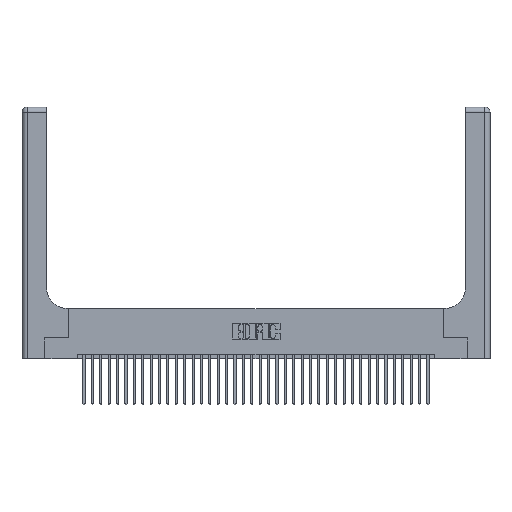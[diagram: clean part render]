
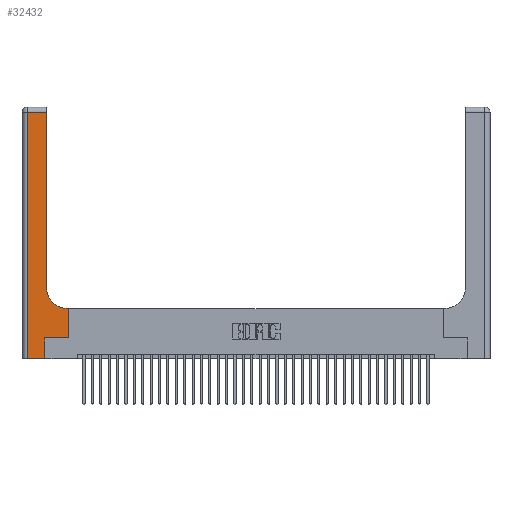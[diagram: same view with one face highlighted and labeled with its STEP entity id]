
A CAD part, top view. The second image highlights one B-rep face of the part: STEP entity #32432.
In plain terms, the highlighted planar face has unit normal (0, 0, 1).
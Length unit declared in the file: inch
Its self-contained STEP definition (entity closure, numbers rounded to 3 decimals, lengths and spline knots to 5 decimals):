
#152 = CARTESIAN_POINT ( 'NONE',  ( 0.5585, 0.6, 0.37 ) ) ;
#202 = LINE ( 'NONE', #612, #22885 ) ;
#358 = EDGE_CURVE ( 'NONE', #30124, #27426, #10339, .T. ) ;
#612 = CARTESIAN_POINT ( 'NONE',  ( 0.269, 0.25, 0.37 ) ) ;
#857 = ORIENTED_EDGE ( 'NONE', *, *, #20001, .T. ) ;
#1382 = FACE_OUTER_BOUND ( 'NONE', #37550, .T. ) ;
#1496 = VERTEX_POINT ( 'NONE', #13183 ) ;
#1788 = CARTESIAN_POINT ( 'NONE',  ( 0.269, 0., 0.37 ) ) ;
#1844 = VERTEX_POINT ( 'NONE', #35211 ) ;
#2411 = VECTOR ( 'NONE', #21373, 39.37008 ) ;
#2478 = VECTOR ( 'NONE', #8937, 39.37008 ) ;
#2539 = CARTESIAN_POINT ( 'NONE',  ( 0.269, 0., 0.37 ) ) ;
#2975 = CARTESIAN_POINT ( 'NONE',  ( 0.06, 0., 0.37 ) ) ;
#3069 = VERTEX_POINT ( 'NONE', #37576 ) ;
#3106 = VERTEX_POINT ( 'NONE', #2539 ) ;
#3187 = VECTOR ( 'NONE', #6990, 39.37008 ) ;
#3831 = EDGE_CURVE ( 'NONE', #27426, #3106, #36082, .T. ) ;
#3844 = VERTEX_POINT ( 'NONE', #32644 ) ;
#3907 = LINE ( 'NONE', #16998, #26511 ) ;
#4087 = ORIENTED_EDGE ( 'NONE', *, *, #19278, .T. ) ;
#5732 = VECTOR ( 'NONE', #6165, 39.37008 ) ;
#6165 = DIRECTION ( 'NONE',  ( 1., 0., 0. ) ) ;
#6990 = DIRECTION ( 'NONE',  ( 0., 1., 0. ) ) ;
#7220 = EDGE_CURVE ( 'NONE', #1844, #3069, #20760, .T. ) ;
#7291 = EDGE_CURVE ( 'NONE', #34413, #14493, #32674, .T. ) ;
#7973 = PLANE ( 'NONE',  #26061 ) ;
#8937 = DIRECTION ( 'NONE',  ( -1., 0., 0. ) ) ;
#9206 = ORIENTED_EDGE ( 'NONE', *, *, #7291, .T. ) ;
#9554 = CARTESIAN_POINT ( 'NONE',  ( 0.06, 3., 0.37 ) ) ;
#10091 = ORIENTED_EDGE ( 'NONE', *, *, #21156, .T. ) ;
#10339 = LINE ( 'NONE', #9554, #2411 ) ;
#10768 = DIRECTION ( 'NONE',  ( 0., 0., -1. ) ) ;
#10820 = CARTESIAN_POINT ( 'NONE',  ( 0., 3., 0.37 ) ) ;
#10959 = DIRECTION ( 'NONE',  ( 0., 0., -1. ) ) ;
#13183 = CARTESIAN_POINT ( 'NONE',  ( 0.269, 0.25, 0.37 ) ) ;
#13193 = DIRECTION ( 'NONE',  ( -1., 0., 0. ) ) ;
#14493 = VERTEX_POINT ( 'NONE', #30005 ) ;
#16546 = DIRECTION ( 'NONE',  ( 0., 1., 0. ) ) ;
#16998 = CARTESIAN_POINT ( 'NONE',  ( 0.5585, 0.25, 0.37 ) ) ;
#17054 = VECTOR ( 'NONE', #13193, 39.37008 ) ;
#18568 = CARTESIAN_POINT ( 'NONE',  ( 0.2915, 3., 0.37 ) ) ;
#18683 = CARTESIAN_POINT ( 'NONE',  ( 0.06, 2.94, 0.37 ) ) ;
#19200 = VECTOR ( 'NONE', #16546, 39.37008 ) ;
#19278 = EDGE_CURVE ( 'NONE', #3106, #1496, #21985, .T. ) ;
#20001 = EDGE_CURVE ( 'NONE', #3844, #34413, #3907, .T. ) ;
#20760 = LINE ( 'NONE', #18568, #3187 ) ;
#21156 = EDGE_CURVE ( 'NONE', #14493, #1844, #33744, .T. ) ;
#21373 = DIRECTION ( 'NONE',  ( 0., -1., 0. ) ) ;
#21985 = LINE ( 'NONE', #1788, #19200 ) ;
#22052 = ORIENTED_EDGE ( 'NONE', *, *, #358, .T. ) ;
#22885 = VECTOR ( 'NONE', #33105, 39.37008 ) ;
#22935 = DIRECTION ( 'NONE',  ( 0., 1., 0. ) ) ;
#23822 = CARTESIAN_POINT ( 'NONE',  ( 0., 0., 0.37 ) ) ;
#24869 = CARTESIAN_POINT ( 'NONE',  ( 0.2915, 0.6, 0.37 ) ) ;
#26061 = AXIS2_PLACEMENT_3D ( 'NONE', #10820, #10959, #31486 ) ;
#26409 = CARTESIAN_POINT ( 'NONE',  ( 0., 2.94, 0.37 ) ) ;
#26511 = VECTOR ( 'NONE', #22935, 39.37008 ) ;
#27426 = VERTEX_POINT ( 'NONE', #2975 ) ;
#28376 = CARTESIAN_POINT ( 'NONE',  ( 0.5415, 0.85, 0.37 ) ) ;
#28524 = ORIENTED_EDGE ( 'NONE', *, *, #29513, .T. ) ;
#29513 = EDGE_CURVE ( 'NONE', #1496, #3844, #202, .T. ) ;
#30005 = CARTESIAN_POINT ( 'NONE',  ( 0.5415, 0.6, 0.37 ) ) ;
#30124 = VERTEX_POINT ( 'NONE', #18683 ) ;
#31306 = DIRECTION ( 'NONE',  ( 1., 0., 0. ) ) ;
#31486 = DIRECTION ( 'NONE',  ( -1., 0., 0. ) ) ;
#31678 = ORIENTED_EDGE ( 'NONE', *, *, #3831, .T. ) ;
#32432 = ADVANCED_FACE ( 'NONE', ( #1382 ), #7973, .F. ) ;
#32644 = CARTESIAN_POINT ( 'NONE',  ( 0.5585, 0.25, 0.37 ) ) ;
#32674 = LINE ( 'NONE', #24869, #17054 ) ;
#33105 = DIRECTION ( 'NONE',  ( 1., 0., 0. ) ) ;
#33744 = CIRCLE ( 'NONE', #35675, 0.25 ) ;
#33832 = LINE ( 'NONE', #26409, #2478 ) ;
#34413 = VERTEX_POINT ( 'NONE', #152 ) ;
#34880 = ORIENTED_EDGE ( 'NONE', *, *, #35710, .T. ) ;
#35211 = CARTESIAN_POINT ( 'NONE',  ( 0.2915, 0.85, 0.37 ) ) ;
#35675 = AXIS2_PLACEMENT_3D ( 'NONE', #28376, #10768, #31306 ) ;
#35710 = EDGE_CURVE ( 'NONE', #3069, #30124, #33832, .T. ) ;
#36082 = LINE ( 'NONE', #23822, #5732 ) ;
#36242 = ORIENTED_EDGE ( 'NONE', *, *, #7220, .T. ) ;
#37550 = EDGE_LOOP ( 'NONE', ( #36242, #34880, #22052, #31678, #4087, #28524, #857, #9206, #10091 ) ) ;
#37576 = CARTESIAN_POINT ( 'NONE',  ( 0.2915, 2.94, 0.37 ) ) ;
